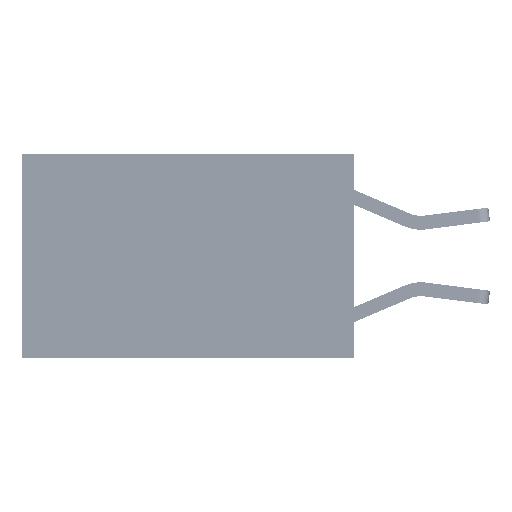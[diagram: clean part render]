
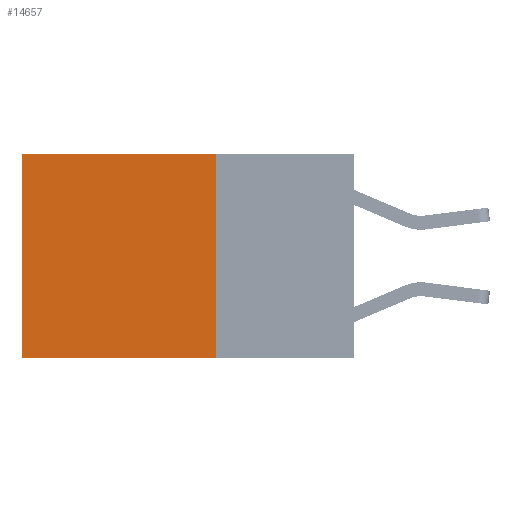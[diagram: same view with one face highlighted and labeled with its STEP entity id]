
A CAD part, left-side view. The second image highlights one B-rep face of the part: STEP entity #14657.
In plain terms, the highlighted planar face has unit normal (-1, 0, 0).
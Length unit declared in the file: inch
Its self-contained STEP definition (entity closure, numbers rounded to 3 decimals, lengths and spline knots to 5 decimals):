
#2 = VERTEX_POINT ( 'NONE', #2273 ) ;
#692 = DIRECTION ( 'NONE',  ( 0., 1., 0. ) ) ;
#772 = DIRECTION ( 'NONE',  ( 0., 0., -1. ) ) ;
#2273 = CARTESIAN_POINT ( 'NONE',  ( 0.2625, 0.25, 0. ) ) ;
#3576 = ORIENTED_EDGE ( 'NONE', *, *, #30430, .T. ) ;
#4838 = LINE ( 'NONE', #25426, #30441 ) ;
#5913 = ORIENTED_EDGE ( 'NONE', *, *, #17072, .F. ) ;
#6514 = FACE_OUTER_BOUND ( 'NONE', #31418, .T. ) ;
#12890 = VERTEX_POINT ( 'NONE', #24016 ) ;
#13011 = LINE ( 'NONE', #27902, #25407 ) ;
#13079 = DIRECTION ( 'NONE',  ( 0., 0., -1. ) ) ;
#13115 = LINE ( 'NONE', #23027, #21243 ) ;
#13149 = PLANE ( 'NONE',  #20518 ) ;
#14657 = ADVANCED_FACE ( 'NONE', ( #6514 ), #13149, .F. ) ;
#15557 = DIRECTION ( 'NONE',  ( 0., 0., -1. ) ) ;
#15624 = DIRECTION ( 'NONE',  ( 1., 0., 0. ) ) ;
#15696 = CARTESIAN_POINT ( 'NONE',  ( 0.2625, 0.25, 0. ) ) ;
#16284 = ORIENTED_EDGE ( 'NONE', *, *, #27454, .F. ) ;
#16393 = VECTOR ( 'NONE', #20665, 39.37008 ) ;
#17072 = EDGE_CURVE ( 'NONE', #2, #28475, #13011, .T. ) ;
#20518 = AXIS2_PLACEMENT_3D ( 'NONE', #27961, #15624, #772 ) ;
#20665 = DIRECTION ( 'NONE',  ( 0., 1., 0. ) ) ;
#21243 = VECTOR ( 'NONE', #15557, 39.37008 ) ;
#21572 = CARTESIAN_POINT ( 'NONE',  ( 0.2625, 0.25, -0.37 ) ) ;
#21877 = EDGE_CURVE ( 'NONE', #12890, #25596, #13115, .T. ) ;
#22974 = LINE ( 'NONE', #15696, #16393 ) ;
#23016 = CARTESIAN_POINT ( 'NONE',  ( 0.2625, 0.6, -0.37 ) ) ;
#23027 = CARTESIAN_POINT ( 'NONE',  ( 0.2625, 0.6, 0. ) ) ;
#24016 = CARTESIAN_POINT ( 'NONE',  ( 0.2625, 0.6, 0. ) ) ;
#25407 = VECTOR ( 'NONE', #13079, 39.37008 ) ;
#25426 = CARTESIAN_POINT ( 'NONE',  ( 0.2625, 0.25, -0.37 ) ) ;
#25596 = VERTEX_POINT ( 'NONE', #23016 ) ;
#27077 = ORIENTED_EDGE ( 'NONE', *, *, #21877, .T. ) ;
#27454 = EDGE_CURVE ( 'NONE', #28475, #25596, #4838, .T. ) ;
#27902 = CARTESIAN_POINT ( 'NONE',  ( 0.2625, 0.25, 0. ) ) ;
#27961 = CARTESIAN_POINT ( 'NONE',  ( 0.2625, 0.25, 0. ) ) ;
#28475 = VERTEX_POINT ( 'NONE', #21572 ) ;
#30430 = EDGE_CURVE ( 'NONE', #2, #12890, #22974, .T. ) ;
#30441 = VECTOR ( 'NONE', #692, 39.37008 ) ;
#31418 = EDGE_LOOP ( 'NONE', ( #27077, #16284, #5913, #3576 ) ) ;
